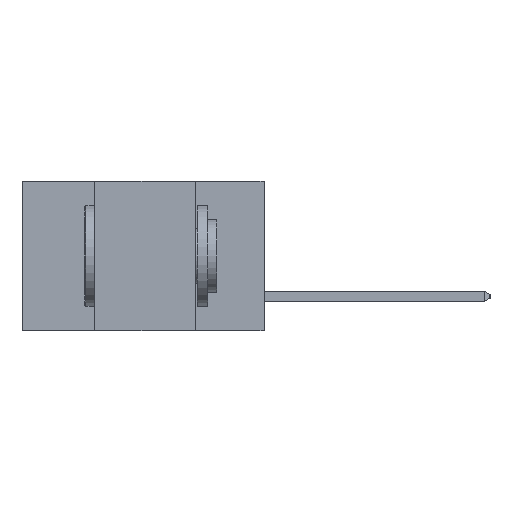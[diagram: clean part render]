
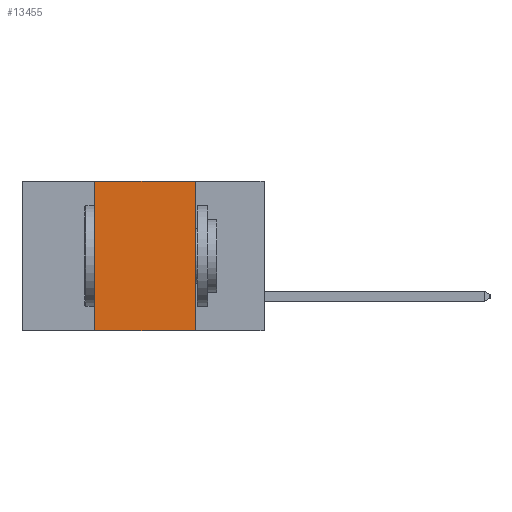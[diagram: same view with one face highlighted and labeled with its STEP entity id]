
A CAD part, left-side view. The second image highlights one B-rep face of the part: STEP entity #13455.
In plain terms, the highlighted planar face has unit normal (-1, 0, 0).
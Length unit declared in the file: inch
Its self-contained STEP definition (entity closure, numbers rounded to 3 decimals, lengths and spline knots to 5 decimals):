
#205 = CARTESIAN_POINT ( 'NONE',  ( 0., 0.17, 0. ) ) ;
#382 = ORIENTED_EDGE ( 'NONE', *, *, #12971, .F. ) ;
#936 = CARTESIAN_POINT ( 'NONE',  ( 0., 0.17, -0.37 ) ) ;
#1171 = CARTESIAN_POINT ( 'NONE',  ( 0., 0.42, -0.37 ) ) ;
#1824 = LINE ( 'NONE', #1171, #12973 ) ;
#2017 = PLANE ( 'NONE',  #8629 ) ;
#2064 = DIRECTION ( 'NONE',  ( 0., 0., -1. ) ) ;
#2125 = ORIENTED_EDGE ( 'NONE', *, *, #12143, .F. ) ;
#2263 = VERTEX_POINT ( 'NONE', #4540 ) ;
#2271 = DIRECTION ( 'NONE',  ( 0., 0., 1. ) ) ;
#2551 = LINE ( 'NONE', #10609, #13626 ) ;
#3628 = VERTEX_POINT ( 'NONE', #205 ) ;
#3764 = VECTOR ( 'NONE', #5125, 39.37008 ) ;
#4540 = CARTESIAN_POINT ( 'NONE',  ( 0., 0.42, -0.37 ) ) ;
#4556 = EDGE_CURVE ( 'NONE', #2263, #12051, #7734, .T. ) ;
#5125 = DIRECTION ( 'NONE',  ( 0., -1., 0. ) ) ;
#5209 = DIRECTION ( 'NONE',  ( 0., -1., 0. ) ) ;
#5522 = ORIENTED_EDGE ( 'NONE', *, *, #9126, .F. ) ;
#5641 = FACE_OUTER_BOUND ( 'NONE', #6720, .T. ) ;
#5771 = CARTESIAN_POINT ( 'NONE',  ( 0., 0.6, -0.37 ) ) ;
#6251 = ORIENTED_EDGE ( 'NONE', *, *, #4556, .T. ) ;
#6502 = DIRECTION ( 'NONE',  ( 0., 0., -1. ) ) ;
#6720 = EDGE_LOOP ( 'NONE', ( #5522, #2125, #382, #6251 ) ) ;
#6880 = CARTESIAN_POINT ( 'NONE',  ( 0., 0.42, 0. ) ) ;
#7584 = CARTESIAN_POINT ( 'NONE',  ( 0., 0.6, 0. ) ) ;
#7698 = VERTEX_POINT ( 'NONE', #6880 ) ;
#7734 = LINE ( 'NONE', #5771, #3764 ) ;
#8629 = AXIS2_PLACEMENT_3D ( 'NONE', #7584, #8655, #2064 ) ;
#8655 = DIRECTION ( 'NONE',  ( 1., 0., 0. ) ) ;
#9126 = EDGE_CURVE ( 'NONE', #3628, #12051, #13537, .T. ) ;
#10470 = CARTESIAN_POINT ( 'NONE',  ( 0., 0.17, -0.37 ) ) ;
#10477 = VECTOR ( 'NONE', #6502, 39.37008 ) ;
#10609 = CARTESIAN_POINT ( 'NONE',  ( 0., 0.6, 0. ) ) ;
#12051 = VERTEX_POINT ( 'NONE', #10470 ) ;
#12143 = EDGE_CURVE ( 'NONE', #7698, #3628, #2551, .T. ) ;
#12971 = EDGE_CURVE ( 'NONE', #2263, #7698, #1824, .T. ) ;
#12973 = VECTOR ( 'NONE', #2271, 39.37008 ) ;
#13455 = ADVANCED_FACE ( 'NONE', ( #5641 ), #2017, .F. ) ;
#13537 = LINE ( 'NONE', #936, #10477 ) ;
#13626 = VECTOR ( 'NONE', #5209, 39.37008 ) ;
